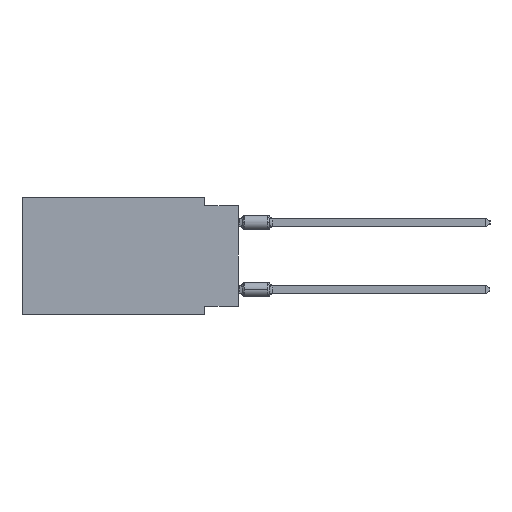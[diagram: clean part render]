
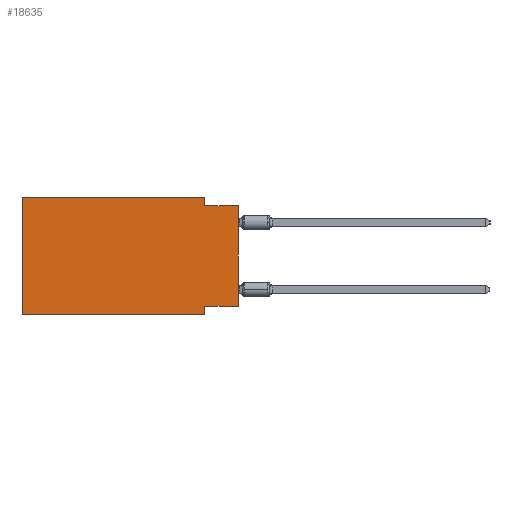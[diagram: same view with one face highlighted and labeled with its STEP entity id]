
A CAD part, left-side view. The second image highlights one B-rep face of the part: STEP entity #18635.
In plain terms, the highlighted planar face has unit normal (-1, 0, 0).
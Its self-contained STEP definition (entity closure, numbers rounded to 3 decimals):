
#1213 = DIRECTION ( 'NONE',  ( 0., 0., 1. ) ) ;
#1914 = EDGE_LOOP ( 'NONE', ( #4696, #45605, #13087, #34732, #16332, #34877, #12269, #10079 ) ) ;
#3528 = EDGE_CURVE ( 'NONE', #49399, #41090, #10823, .T. ) ;
#3600 = PLANE ( 'NONE',  #38986 ) ;
#4226 = VECTOR ( 'NONE', #33088, 1000. ) ;
#4696 = ORIENTED_EDGE ( 'NONE', *, *, #50029, .T. ) ;
#5279 = VECTOR ( 'NONE', #42887, 1000. ) ;
#5391 = VERTEX_POINT ( 'NONE', #9099 ) ;
#6486 = LINE ( 'NONE', #52405, #27603 ) ;
#6941 = EDGE_CURVE ( 'NONE', #41090, #22173, #16667, .T. ) ;
#8325 = CARTESIAN_POINT ( 'NONE',  ( 0., 16.383, 0. ) ) ;
#8541 = CARTESIAN_POINT ( 'NONE',  ( 0., 16.383, 0. ) ) ;
#9099 = CARTESIAN_POINT ( 'NONE',  ( 0., 16.383, -8.89 ) ) ;
#10079 = ORIENTED_EDGE ( 'NONE', *, *, #46769, .F. ) ;
#10823 = LINE ( 'NONE', #30917, #5279 ) ;
#11120 = VECTOR ( 'NONE', #30871, 1000. ) ;
#11465 = CARTESIAN_POINT ( 'NONE',  ( 0., 16.383, 0. ) ) ;
#11500 = DIRECTION ( 'NONE',  ( 0., 0., -1. ) ) ;
#12269 = ORIENTED_EDGE ( 'NONE', *, *, #26453, .F. ) ;
#13087 = ORIENTED_EDGE ( 'NONE', *, *, #6941, .F. ) ;
#14542 = CARTESIAN_POINT ( 'NONE',  ( 0., 0., -8.255 ) ) ;
#14549 = CARTESIAN_POINT ( 'NONE',  ( 0., 2.54, -0.635 ) ) ;
#14713 = VECTOR ( 'NONE', #11500, 1000. ) ;
#15543 = CARTESIAN_POINT ( 'NONE',  ( 0., 0., 0. ) ) ;
#16332 = ORIENTED_EDGE ( 'NONE', *, *, #47406, .F. ) ;
#16667 = LINE ( 'NONE', #36737, #14713 ) ;
#17540 = VERTEX_POINT ( 'NONE', #52219 ) ;
#18293 = VECTOR ( 'NONE', #39698, 1000. ) ;
#18635 = ADVANCED_FACE ( 'NONE', ( #36963 ), #3600, .F. ) ;
#19877 = DIRECTION ( 'NONE',  ( 0., 0., -1. ) ) ;
#22173 = VERTEX_POINT ( 'NONE', #14549 ) ;
#22971 = VERTEX_POINT ( 'NONE', #38859 ) ;
#23596 = DIRECTION ( 'NONE',  ( 0., 0., -1. ) ) ;
#24147 = VECTOR ( 'NONE', #1213, 1000. ) ;
#26453 = EDGE_CURVE ( 'NONE', #30134, #17540, #6486, .T. ) ;
#26496 = EDGE_CURVE ( 'NONE', #5391, #17540, #53490, .T. ) ;
#27081 = CARTESIAN_POINT ( 'NONE',  ( 0., 0., -8.255 ) ) ;
#27603 = VECTOR ( 'NONE', #23596, 1000. ) ;
#28102 = VERTEX_POINT ( 'NONE', #14542 ) ;
#29066 = EDGE_CURVE ( 'NONE', #22173, #22971, #34192, .T. ) ;
#29574 = DIRECTION ( 'NONE',  ( 0., -1., 0. ) ) ;
#30134 = VERTEX_POINT ( 'NONE', #52438 ) ;
#30871 = DIRECTION ( 'NONE',  ( 0., 1., 0. ) ) ;
#30917 = CARTESIAN_POINT ( 'NONE',  ( 0., 16.383, 0. ) ) ;
#32495 = CARTESIAN_POINT ( 'NONE',  ( 0., 2.54, 0. ) ) ;
#33088 = DIRECTION ( 'NONE',  ( 0., -1., 0. ) ) ;
#34184 = VECTOR ( 'NONE', #29574, 1000. ) ;
#34192 = LINE ( 'NONE', #38270, #34184 ) ;
#34732 = ORIENTED_EDGE ( 'NONE', *, *, #3528, .F. ) ;
#34877 = ORIENTED_EDGE ( 'NONE', *, *, #26496, .T. ) ;
#36737 = CARTESIAN_POINT ( 'NONE',  ( 0., 2.54, 0. ) ) ;
#36963 = FACE_OUTER_BOUND ( 'NONE', #1914, .T. ) ;
#38270 = CARTESIAN_POINT ( 'NONE',  ( 0., 0., -0.635 ) ) ;
#38859 = CARTESIAN_POINT ( 'NONE',  ( 0., 0., -0.635 ) ) ;
#38986 = AXIS2_PLACEMENT_3D ( 'NONE', #11465, #53583, #19877 ) ;
#39295 = LINE ( 'NONE', #27081, #11120 ) ;
#39698 = DIRECTION ( 'NONE',  ( 0., 0., 1. ) ) ;
#41090 = VERTEX_POINT ( 'NONE', #32495 ) ;
#41919 = LINE ( 'NONE', #8541, #24147 ) ;
#42887 = DIRECTION ( 'NONE',  ( 0., -1., 0. ) ) ;
#44588 = LINE ( 'NONE', #15543, #18293 ) ;
#45605 = ORIENTED_EDGE ( 'NONE', *, *, #29066, .F. ) ;
#46769 = EDGE_CURVE ( 'NONE', #28102, #30134, #39295, .T. ) ;
#47406 = EDGE_CURVE ( 'NONE', #5391, #49399, #41919, .T. ) ;
#49399 = VERTEX_POINT ( 'NONE', #8325 ) ;
#50029 = EDGE_CURVE ( 'NONE', #28102, #22971, #44588, .T. ) ;
#52219 = CARTESIAN_POINT ( 'NONE',  ( 0., 2.54, -8.89 ) ) ;
#52405 = CARTESIAN_POINT ( 'NONE',  ( 0., 2.54, -8.89 ) ) ;
#52438 = CARTESIAN_POINT ( 'NONE',  ( 0., 2.54, -8.255 ) ) ;
#53221 = CARTESIAN_POINT ( 'NONE',  ( 0., 16.383, -8.89 ) ) ;
#53490 = LINE ( 'NONE', #53221, #4226 ) ;
#53583 = DIRECTION ( 'NONE',  ( 1., 0., 0. ) ) ;
